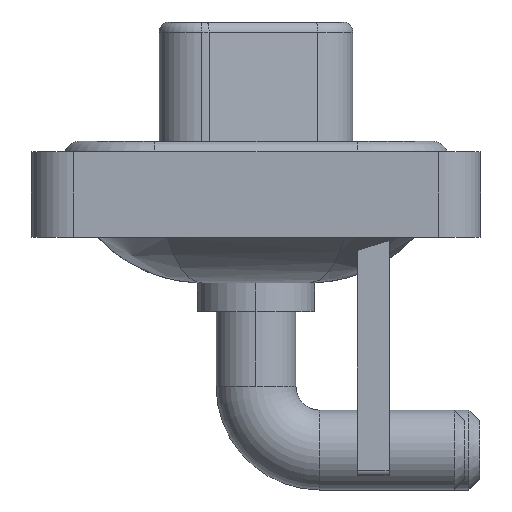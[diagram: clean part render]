
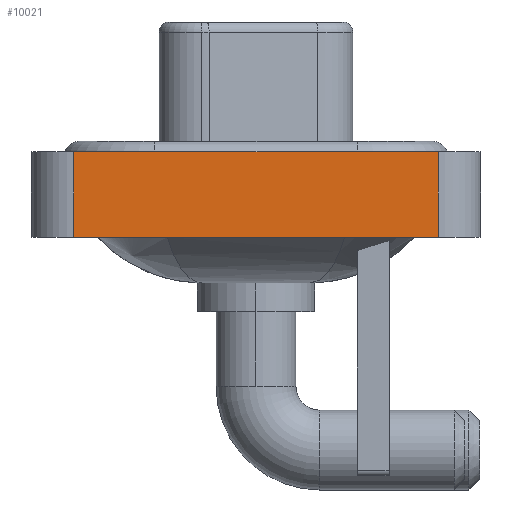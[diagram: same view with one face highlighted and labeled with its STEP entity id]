
A CAD part, left-side view. The second image highlights one B-rep face of the part: STEP entity #10021.
In plain terms, the highlighted planar face has unit normal (-1, 0, 0).
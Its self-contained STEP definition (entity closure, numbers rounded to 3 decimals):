
#630 = ORIENTED_EDGE ( 'NONE', *, *, #12739, .F. ) ;
#1271 = CARTESIAN_POINT ( 'NONE',  ( -7.3, 8.55, 0.4 ) ) ;
#3131 = ORIENTED_EDGE ( 'NONE', *, *, #19252, .T. ) ;
#3341 = CARTESIAN_POINT ( 'NONE',  ( -7.3, -8.55, -3.6 ) ) ;
#3444 = CARTESIAN_POINT ( 'NONE',  ( -7.3, -8.55, -3.6 ) ) ;
#4857 = PLANE ( 'NONE',  #9536 ) ;
#4991 = LINE ( 'NONE', #9195, #5201 ) ;
#5057 = DIRECTION ( 'NONE',  ( -1., 0., 0. ) ) ;
#5201 = VECTOR ( 'NONE', #6153, 1000. ) ;
#6153 = DIRECTION ( 'NONE',  ( 0., -1., 0. ) ) ;
#6381 = DIRECTION ( 'NONE',  ( 0., 0., 1. ) ) ;
#7640 = CARTESIAN_POINT ( 'NONE',  ( -7.3, -8.55, -3.6 ) ) ;
#8026 = LINE ( 'NONE', #7640, #18642 ) ;
#8183 = EDGE_CURVE ( 'NONE', #18944, #18965, #17285, .T. ) ;
#9195 = CARTESIAN_POINT ( 'NONE',  ( -7.3, -8.55, 0.4 ) ) ;
#9272 = EDGE_LOOP ( 'NONE', ( #3131, #630, #15060, #16750 ) ) ;
#9474 = EDGE_CURVE ( 'NONE', #18944, #19150, #12204, .T. ) ;
#9536 = AXIS2_PLACEMENT_3D ( 'NONE', #3444, #5057, #6381 ) ;
#9627 = DIRECTION ( 'NONE',  ( 0., -1., 0. ) ) ;
#10021 = ADVANCED_FACE ( 'NONE', ( #12990 ), #4857, .T. ) ;
#12107 = VECTOR ( 'NONE', #17026, 1000. ) ;
#12203 = DIRECTION ( 'NONE',  ( 0., 0., 1. ) ) ;
#12204 = LINE ( 'NONE', #18749, #12107 ) ;
#12739 = EDGE_CURVE ( 'NONE', #19150, #17082, #4991, .T. ) ;
#12990 = FACE_OUTER_BOUND ( 'NONE', #9272, .T. ) ;
#14352 = CARTESIAN_POINT ( 'NONE',  ( -7.3, -8.55, -3.6 ) ) ;
#15060 = ORIENTED_EDGE ( 'NONE', *, *, #9474, .F. ) ;
#15669 = VECTOR ( 'NONE', #9627, 1000. ) ;
#15996 = CARTESIAN_POINT ( 'NONE',  ( -7.3, -8.55, 0.4 ) ) ;
#16750 = ORIENTED_EDGE ( 'NONE', *, *, #8183, .T. ) ;
#17026 = DIRECTION ( 'NONE',  ( 0., 0., 1. ) ) ;
#17082 = VERTEX_POINT ( 'NONE', #15996 ) ;
#17285 = LINE ( 'NONE', #3341, #15669 ) ;
#18642 = VECTOR ( 'NONE', #12203, 1000. ) ;
#18749 = CARTESIAN_POINT ( 'NONE',  ( -7.3, 8.55, -3.6 ) ) ;
#18944 = VERTEX_POINT ( 'NONE', #19459 ) ;
#18965 = VERTEX_POINT ( 'NONE', #14352 ) ;
#19150 = VERTEX_POINT ( 'NONE', #1271 ) ;
#19252 = EDGE_CURVE ( 'NONE', #18965, #17082, #8026, .T. ) ;
#19459 = CARTESIAN_POINT ( 'NONE',  ( -7.3, 8.55, -3.6 ) ) ;
